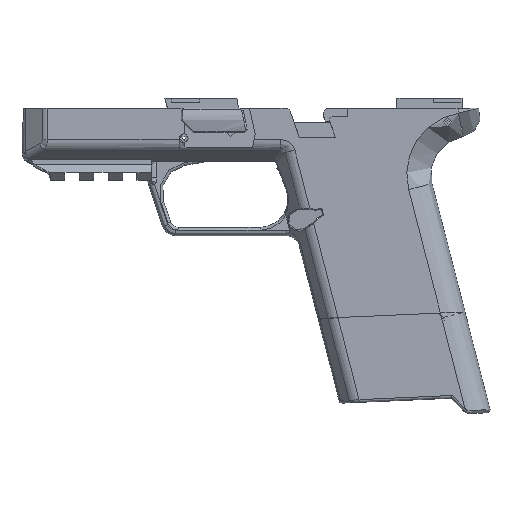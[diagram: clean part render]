
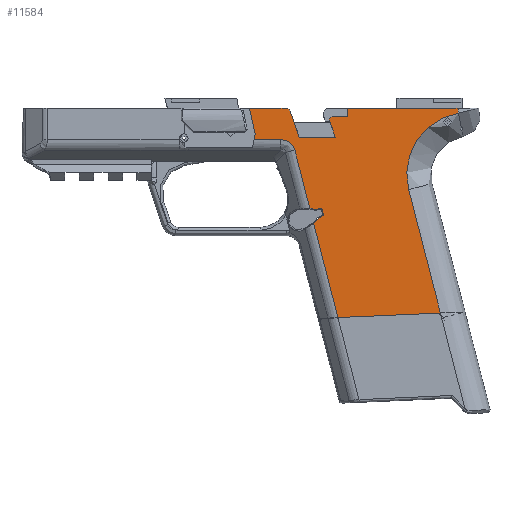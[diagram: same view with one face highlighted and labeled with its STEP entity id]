
A CAD part, left-side view. The second image highlights one B-rep face of the part: STEP entity #11584.
In plain terms, the highlighted face is planar.
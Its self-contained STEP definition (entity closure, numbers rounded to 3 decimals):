
#127=ELLIPSE('',#12485,10.693,7.);
#755=PLANE('',#12480);
#1174=FACE_OUTER_BOUND('',#1836,.T.);
#1836=EDGE_LOOP('',(#8901,#8902,#8903,#8904,#8905,#8906,#8907,#8908,#8909,
#8910,#8911,#8912,#8913,#8914,#8915,#8916,#8917,#8918,#8919,#8920,#8921,
#8922,#8923,#8924,#8925));
#2699=LINE('',#18610,#3804);
#2705=LINE('',#18620,#3810);
#2709=LINE('',#18628,#3814);
#2720=LINE('',#18687,#3825);
#2746=LINE('',#18752,#3851);
#2747=LINE('',#18754,#3852);
#2748=LINE('',#18756,#3853);
#2749=LINE('',#18762,#3854);
#2750=LINE('',#18764,#3855);
#2751=LINE('',#18766,#3856);
#2752=LINE('',#18770,#3857);
#2753=LINE('',#18772,#3858);
#2754=LINE('',#18774,#3859);
#2755=LINE('',#18778,#3860);
#2756=LINE('',#18780,#3861);
#2757=LINE('',#18782,#3862);
#2758=LINE('',#18784,#3863);
#2759=LINE('',#18787,#3864);
#3804=VECTOR('',#14300,10.);
#3810=VECTOR('',#14310,10.);
#3814=VECTOR('',#14318,10.);
#3825=VECTOR('',#14351,10.);
#3851=VECTOR('',#14411,10.);
#3852=VECTOR('',#14412,10.);
#3853=VECTOR('',#14413,10.);
#3854=VECTOR('',#14418,10.);
#3855=VECTOR('',#14419,10.);
#3856=VECTOR('',#14420,10.);
#3857=VECTOR('',#14423,10.);
#3858=VECTOR('',#14424,10.);
#3859=VECTOR('',#14425,10.);
#3860=VECTOR('',#14428,10.);
#3861=VECTOR('',#14429,10.);
#3862=VECTOR('',#14430,10.);
#3863=VECTOR('',#14431,10.);
#3864=VECTOR('',#14434,10.);
#4576=CIRCLE('',#12454,2.822);
#4577=CIRCLE('',#12458,2.822);
#4579=CIRCLE('',#12481,22.475);
#4580=CIRCLE('',#12482,7.5);
#4581=CIRCLE('',#12483,1.);
#4582=CIRCLE('',#12484,2.);
#5198=VERTEX_POINT('',#18607);
#5199=VERTEX_POINT('',#18609);
#5201=VERTEX_POINT('',#18618);
#5203=VERTEX_POINT('',#18627);
#5206=VERTEX_POINT('',#18641);
#5208=VERTEX_POINT('',#18648);
#5218=VERTEX_POINT('',#18685);
#5240=VERTEX_POINT('',#18751);
#5241=VERTEX_POINT('',#18753);
#5242=VERTEX_POINT('',#18755);
#5243=VERTEX_POINT('',#18757);
#5244=VERTEX_POINT('',#18759);
#5245=VERTEX_POINT('',#18761);
#5246=VERTEX_POINT('',#18763);
#5247=VERTEX_POINT('',#18765);
#5248=VERTEX_POINT('',#18767);
#5249=VERTEX_POINT('',#18769);
#5250=VERTEX_POINT('',#18771);
#5251=VERTEX_POINT('',#18773);
#5252=VERTEX_POINT('',#18775);
#5253=VERTEX_POINT('',#18777);
#5254=VERTEX_POINT('',#18779);
#5255=VERTEX_POINT('',#18781);
#5256=VERTEX_POINT('',#18783);
#5257=VERTEX_POINT('',#18785);
#6515=EDGE_CURVE('',#5199,#5198,#2699,.T.);
#6521=EDGE_CURVE('',#5198,#5201,#2705,.T.);
#6525=EDGE_CURVE('',#5203,#5199,#2709,.T.);
#6529=EDGE_CURVE('',#5201,#5206,#4576,.T.);
#6532=EDGE_CURVE('',#5208,#5203,#4577,.T.);
#6546=EDGE_CURVE('',#5206,#5218,#2720,.T.);
#6579=EDGE_CURVE('',#5240,#5218,#2746,.T.);
#6580=EDGE_CURVE('',#5241,#5240,#2747,.T.);
#6581=EDGE_CURVE('',#5242,#5241,#2748,.T.);
#6582=EDGE_CURVE('',#5243,#5242,#4579,.T.);
#6583=EDGE_CURVE('',#5244,#5243,#4580,.T.);
#6584=EDGE_CURVE('',#5244,#5245,#2749,.T.);
#6585=EDGE_CURVE('',#5245,#5246,#2750,.F.);
#6586=EDGE_CURVE('',#5246,#5247,#2751,.T.);
#6587=EDGE_CURVE('',#5248,#5247,#4581,.T.);
#6588=EDGE_CURVE('',#5248,#5249,#2752,.F.);
#6589=EDGE_CURVE('',#5249,#5250,#2753,.T.);
#6590=EDGE_CURVE('',#5250,#5251,#2754,.F.);
#6591=EDGE_CURVE('',#5252,#5251,#4582,.T.);
#6592=EDGE_CURVE('',#5252,#5253,#2755,.T.);
#6593=EDGE_CURVE('',#5253,#5254,#2756,.T.);
#6594=EDGE_CURVE('',#5254,#5255,#2757,.T.);
#6595=EDGE_CURVE('',#5256,#5255,#2758,.T.);
#6596=EDGE_CURVE('',#5257,#5256,#127,.T.);
#6597=EDGE_CURVE('',#5208,#5257,#2759,.T.);
#8901=ORIENTED_EDGE('',*,*,#6532,.T.);
#8902=ORIENTED_EDGE('',*,*,#6525,.T.);
#8903=ORIENTED_EDGE('',*,*,#6515,.T.);
#8904=ORIENTED_EDGE('',*,*,#6521,.T.);
#8905=ORIENTED_EDGE('',*,*,#6529,.T.);
#8906=ORIENTED_EDGE('',*,*,#6546,.T.);
#8907=ORIENTED_EDGE('',*,*,#6579,.F.);
#8908=ORIENTED_EDGE('',*,*,#6580,.F.);
#8909=ORIENTED_EDGE('',*,*,#6581,.F.);
#8910=ORIENTED_EDGE('',*,*,#6582,.F.);
#8911=ORIENTED_EDGE('',*,*,#6583,.F.);
#8912=ORIENTED_EDGE('',*,*,#6584,.T.);
#8913=ORIENTED_EDGE('',*,*,#6585,.T.);
#8914=ORIENTED_EDGE('',*,*,#6586,.T.);
#8915=ORIENTED_EDGE('',*,*,#6587,.F.);
#8916=ORIENTED_EDGE('',*,*,#6588,.T.);
#8917=ORIENTED_EDGE('',*,*,#6589,.T.);
#8918=ORIENTED_EDGE('',*,*,#6590,.T.);
#8919=ORIENTED_EDGE('',*,*,#6591,.F.);
#8920=ORIENTED_EDGE('',*,*,#6592,.T.);
#8921=ORIENTED_EDGE('',*,*,#6593,.T.);
#8922=ORIENTED_EDGE('',*,*,#6594,.T.);
#8923=ORIENTED_EDGE('',*,*,#6595,.F.);
#8924=ORIENTED_EDGE('',*,*,#6596,.F.);
#8925=ORIENTED_EDGE('',*,*,#6597,.F.);
#11584=ADVANCED_FACE('',(#1174),#755,.F.);
#12454=AXIS2_PLACEMENT_3D('',#18643,#14323,#14324);
#12458=AXIS2_PLACEMENT_3D('',#18649,#14331,#14332);
#12480=AXIS2_PLACEMENT_3D('',#18750,#14409,#14410);
#12481=AXIS2_PLACEMENT_3D('',#18758,#14414,#14415);
#12482=AXIS2_PLACEMENT_3D('',#18760,#14416,#14417);
#12483=AXIS2_PLACEMENT_3D('',#18768,#14421,#14422);
#12484=AXIS2_PLACEMENT_3D('',#18776,#14426,#14427);
#12485=AXIS2_PLACEMENT_3D('',#18786,#14432,#14433);
#14300=DIRECTION('',(0.,-0.323,0.947));
#14310=DIRECTION('',(0.,0.866,0.5));
#14318=DIRECTION('',(0.,-0.991,-0.133));
#14323=DIRECTION('center_axis',(-1.,0.,0.));
#14324=DIRECTION('ref_axis',(0.,-0.56,0.828));
#14331=DIRECTION('center_axis',(-1.,0.,0.));
#14332=DIRECTION('ref_axis',(0.,-0.504,-0.864));
#14351=DIRECTION('',(0.,0.828,0.56));
#14409=DIRECTION('center_axis',(-1.,0.,0.));
#14410=DIRECTION('ref_axis',(0.,1.,0.));
#14411=DIRECTION('',(0.,0.249,-0.969));
#14412=DIRECTION('',(0.,0.999,0.044));
#14413=DIRECTION('',(0.,-0.249,0.969));
#14414=DIRECTION('center_axis',(1.,0.,0.));
#14415=DIRECTION('ref_axis',(0.,0.,
1.));
#14416=DIRECTION('center_axis',(1.,0.,0.));
#14417=DIRECTION('ref_axis',(0.,-0.97,-0.244));
#14418=DIRECTION('',(0.,1.,0.));
#14419=DIRECTION('',(0.,0.,-1.));
#14420=DIRECTION('',(0.,1.,0.));
#14421=DIRECTION('center_axis',(-1.,0.,0.));
#14422=DIRECTION('ref_axis',(0.,0.817,-0.576));
#14423=DIRECTION('',(0.,0.336,-0.942));
#14424=DIRECTION('',(0.,1.,0.));
#14425=DIRECTION('',(0.,-0.336,0.942));
#14426=DIRECTION('center_axis',(-1.,0.,0.));
#14427=DIRECTION('ref_axis',(0.,-0.576,-0.817));
#14428=DIRECTION('',(0.,1.,0.));
#14429=DIRECTION('',(0.,-0.21,0.978));
#14430=DIRECTION('',(0.,0.21,0.978));
#14431=DIRECTION('',(0.,1.,0.));
#14432=DIRECTION('center_axis',(1.,0.,0.));
#14433=DIRECTION('ref_axis',(0.,-0.714,-0.7));
#14434=DIRECTION('',(0.,0.249,-0.969));
#18607=CARTESIAN_POINT('',(22.175,-30.382,31.415));
#18609=CARTESIAN_POINT('',(22.175,-29.529,28.913));
#18610=CARTESIAN_POINT('',(22.175,-24.222,13.336));
#18618=CARTESIAN_POINT('',(22.175,-28.028,32.774));
#18620=CARTESIAN_POINT('',(22.175,-27.537,33.057));
#18627=CARTESIAN_POINT('',(22.175,-26.835,29.274));
#18628=CARTESIAN_POINT('',(22.175,-18.345,30.412));
#18641=CARTESIAN_POINT('',(22.175,-26.995,34.049));
#18643=CARTESIAN_POINT('Origin',(22.175,-25.413,31.712));
#18648=CARTESIAN_POINT('',(22.175,-25.244,28.895));
#18649=CARTESIAN_POINT('Origin',(22.175,-25.413,31.712));
#18685=CARTESIAN_POINT('',(22.175,-26.632,34.294));
#18687=CARTESIAN_POINT('',(22.175,-27.16,33.937));
#18750=CARTESIAN_POINT('Origin',(22.175,-5.921,2.186));
#18751=CARTESIAN_POINT('',(22.175,-35.447,68.587));
#18752=CARTESIAN_POINT('',(22.175,-24.659,26.619));
#18753=CARTESIAN_POINT('',(22.175,-72.722,66.935));
#18754=CARTESIAN_POINT('',(22.175,-38.785,68.439));
#18755=CARTESIAN_POINT('',(22.175,-61.184,22.049));
#18756=CARTESIAN_POINT('',(22.175,-73.103,68.418));
#18757=CARTESIAN_POINT('',(22.175,-79.332,-5.728));
#18758=CARTESIAN_POINT('Origin',(22.175,-82.951,16.453));
#18759=CARTESIAN_POINT('',(22.175,-79.106,-7.556));
#18760=CARTESIAN_POINT('Origin',(22.175,-86.606,-7.556));
#18761=CARTESIAN_POINT('',(22.175,-38.774,-7.556));
#18762=CARTESIAN_POINT('',(22.175,-82.951,-7.556));
#18763=CARTESIAN_POINT('',(22.175,-38.774,-4.331));
#18764=CARTESIAN_POINT('',(22.175,-38.774,-2.685));
#18765=CARTESIAN_POINT('',(22.175,-33.316,-4.331));
#18766=CARTESIAN_POINT('',(22.175,-18.598,-4.331));
#18767=CARTESIAN_POINT('',(22.175,-32.374,-2.995));
#18768=CARTESIAN_POINT('Origin',(22.175,-33.316,-3.331));
#18769=CARTESIAN_POINT('',(22.175,-34.514,3.));
#18770=CARTESIAN_POINT('',(22.175,-30.976,-6.913));
#18771=CARTESIAN_POINT('',(22.175,-21.407,3.));
#18772=CARTESIAN_POINT('',(22.175,-21.764,3.));
#18773=CARTESIAN_POINT('',(22.175,-18.114,-6.228));
#18774=CARTESIAN_POINT('',(22.175,-19.552,-2.199));
#18775=CARTESIAN_POINT('',(22.175,-16.23,-7.556));
#18776=CARTESIAN_POINT('Origin',(22.175,-16.23,-5.556));
#18777=CARTESIAN_POINT('',(22.175,-3.3,-7.556));
#18778=CARTESIAN_POINT('',(22.175,-84.951,-7.556));
#18779=CARTESIAN_POINT('',(22.175,-5.389,2.186));
#18780=CARTESIAN_POINT('',(22.175,-4.356,-2.63));
#18781=CARTESIAN_POINT('',(22.175,-5.025,3.884));
#18782=CARTESIAN_POINT('',(22.175,-5.4,2.132));
#18783=CARTESIAN_POINT('',(22.175,-14.536,3.884));
#18784=CARTESIAN_POINT('',(22.175,35.814,3.884));
#18785=CARTESIAN_POINT('',(22.175,-19.783,7.651));
#18786=CARTESIAN_POINT('Origin',(22.175,-10.907,12.884));
#18787=CARTESIAN_POINT('',(22.175,-24.659,26.619));
